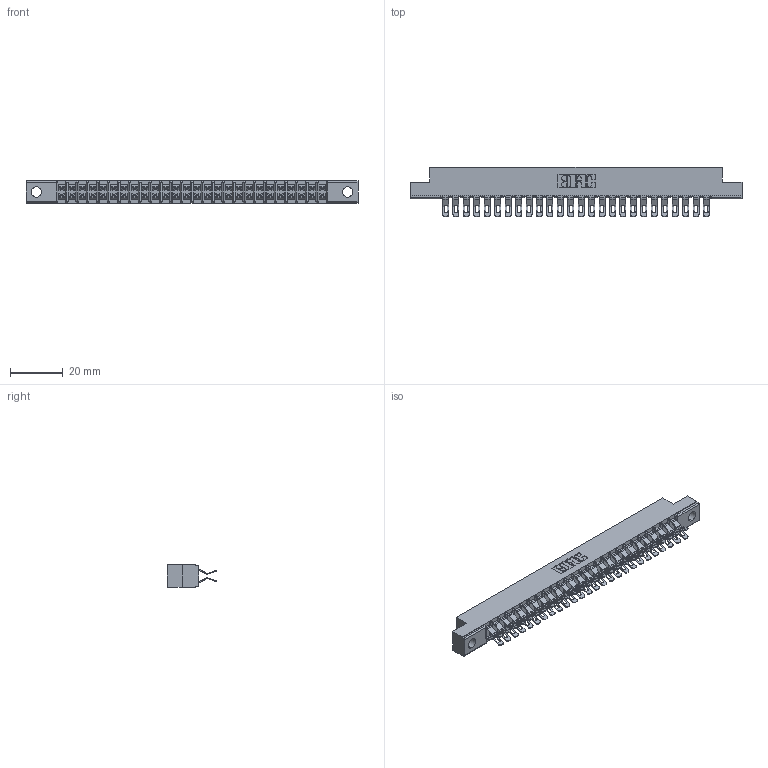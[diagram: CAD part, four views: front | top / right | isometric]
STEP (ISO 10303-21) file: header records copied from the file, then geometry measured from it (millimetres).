
FILE_DESCRIPTION (( 'STEP AP203' ), '1' );
FILE_NAME ('357-052-555-204.STEP', '2018-08-11T15:58:09', ( '' ), ( '' ), 'SwSTEP 2.0', 'SolidWorks 2016', '' );
FILE_SCHEMA (( 'CONFIG_CONTROL_DESIGN' ));
Length unit declared in the file: inch
Products named in the file (3): 357-052-555-204; 307 Part_.156 Dia Mounting Holes; 307-290-001_555
Assembly tree (53 placements, depth 2):
  357-052-555-204
    307 Part_.156 Dia Mounting Holes
    307-290-001_555  x52
Bounding box: 126.03 x 18.75 x 8.71 mm (x, y, z)
Volume: 8292.6 mm3; surface area: 15599.4 mm2
Topology: 53 solids, 53 shells, 3331 faces, 9771 edges, 6370 vertices
Faces by surface type: plane 1852, cylinder 1425, sphere 54
Entity records: 26049 total; most frequent: CARTESIAN_POINT 4276, ORIENTED_EDGE 4236, DIRECTION 4194, EDGE_CURVE 2118, LINE 1614, VECTOR 1614, VERTEX_POINT 1372, AXIS2_PLACEMENT_3D 1290
